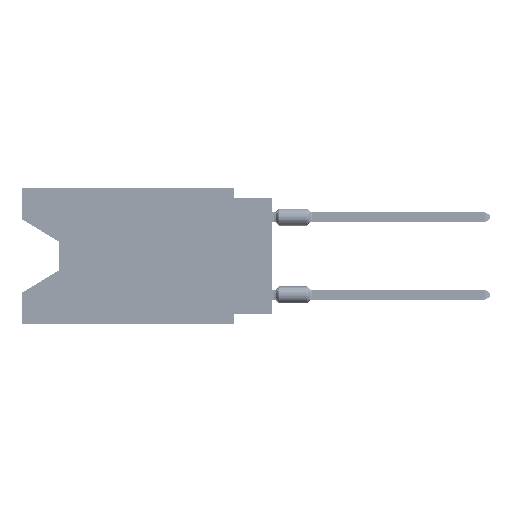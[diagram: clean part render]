
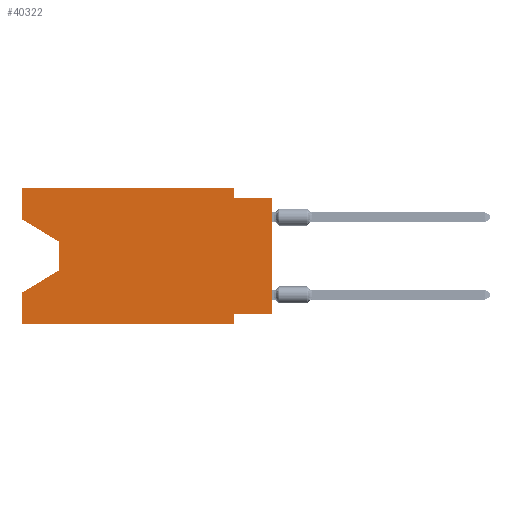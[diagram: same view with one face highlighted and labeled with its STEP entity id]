
A CAD part, left-side view. The second image highlights one B-rep face of the part: STEP entity #40322.
In plain terms, the highlighted planar face has unit normal (-1, 0, 0).
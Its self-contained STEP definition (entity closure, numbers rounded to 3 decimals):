
#5872 = VECTOR ( 'NONE', #108346, 1000. ) ;
#6425 = VECTOR ( 'NONE', #30490, 1000. ) ;
#6697 = ORIENTED_EDGE ( 'NONE', *, *, #8738, .T. ) ;
#8738 = EDGE_CURVE ( 'NONE', #48534, #78207, #15025, .T. ) ;
#10469 = LINE ( 'NONE', #19357, #81993 ) ;
#10480 = LINE ( 'NONE', #92791, #23293 ) ;
#11209 = ORIENTED_EDGE ( 'NONE', *, *, #109093, .F. ) ;
#12362 = CARTESIAN_POINT ( 'NONE',  ( 0., 13.97, -5.385 ) ) ;
#12400 = EDGE_CURVE ( 'NONE', #58064, #49808, #10480, .T. ) ;
#12422 = PLANE ( 'NONE',  #38660 ) ;
#14080 = CARTESIAN_POINT ( 'NONE',  ( 0., 16.383, 0. ) ) ;
#15025 = LINE ( 'NONE', #51156, #77540 ) ;
#15760 = EDGE_CURVE ( 'NONE', #78986, #49808, #52710, .T. ) ;
#15952 = CARTESIAN_POINT ( 'NONE',  ( 0., 0., -0.635 ) ) ;
#19357 = CARTESIAN_POINT ( 'NONE',  ( 0., 16.383, -2.038 ) ) ;
#20990 = ORIENTED_EDGE ( 'NONE', *, *, #60506, .F. ) ;
#23271 = ORIENTED_EDGE ( 'NONE', *, *, #80783, .F. ) ;
#23293 = VECTOR ( 'NONE', #46021, 1000. ) ;
#23773 = CARTESIAN_POINT ( 'NONE',  ( 0., 2.54, -8.255 ) ) ;
#24682 = DIRECTION ( 'NONE',  ( 0., 0., -1. ) ) ;
#24844 = CARTESIAN_POINT ( 'NONE',  ( 0., 16.383, 0. ) ) ;
#27945 = CARTESIAN_POINT ( 'NONE',  ( 0., 16.383, -8.89 ) ) ;
#30178 = ORIENTED_EDGE ( 'NONE', *, *, #110683, .T. ) ;
#30490 = DIRECTION ( 'NONE',  ( 0., 0., 1. ) ) ;
#30804 = CARTESIAN_POINT ( 'NONE',  ( 0., 16.383, 0. ) ) ;
#31590 = CARTESIAN_POINT ( 'NONE',  ( 0., 0., -0.635 ) ) ;
#32612 = CARTESIAN_POINT ( 'NONE',  ( 0., 13.97, -3.505 ) ) ;
#34746 = CARTESIAN_POINT ( 'NONE',  ( 0., 2.54, -0.635 ) ) ;
#35360 = CARTESIAN_POINT ( 'NONE',  ( 0., 16.383, 0. ) ) ;
#36560 = ORIENTED_EDGE ( 'NONE', *, *, #15760, .T. ) ;
#38660 = AXIS2_PLACEMENT_3D ( 'NONE', #48562, #68081, #59774 ) ;
#39693 = DIRECTION ( 'NONE',  ( 0., 0., 1. ) ) ;
#40322 = ADVANCED_FACE ( 'NONE', ( #40840 ), #12422, .F. ) ;
#40840 = FACE_OUTER_BOUND ( 'NONE', #113169, .T. ) ;
#43012 = VERTEX_POINT ( 'NONE', #34746 ) ;
#46021 = DIRECTION ( 'NONE',  ( 0., 0., -1. ) ) ;
#48250 = CARTESIAN_POINT ( 'NONE',  ( 0., 0., 0. ) ) ;
#48318 = ORIENTED_EDGE ( 'NONE', *, *, #92590, .T. ) ;
#48534 = VERTEX_POINT ( 'NONE', #12362 ) ;
#48562 = CARTESIAN_POINT ( 'NONE',  ( 0., 16.383, 0. ) ) ;
#48840 = LINE ( 'NONE', #48250, #6425 ) ;
#49808 = VERTEX_POINT ( 'NONE', #74140 ) ;
#51156 = CARTESIAN_POINT ( 'NONE',  ( 0., 13.97, -5.385 ) ) ;
#51755 = VECTOR ( 'NONE', #105972, 1000. ) ;
#52127 = CARTESIAN_POINT ( 'NONE',  ( 0., 16.383, -8.89 ) ) ;
#52710 = LINE ( 'NONE', #52127, #5872 ) ;
#55257 = VERTEX_POINT ( 'NONE', #88726 ) ;
#56885 = LINE ( 'NONE', #30804, #67182 ) ;
#58064 = VERTEX_POINT ( 'NONE', #23773 ) ;
#59415 = EDGE_CURVE ( 'NONE', #86997, #58064, #99359, .T. ) ;
#59774 = DIRECTION ( 'NONE',  ( 0., 0., -1. ) ) ;
#59967 = VECTOR ( 'NONE', #69463, 1000. ) ;
#60506 = EDGE_CURVE ( 'NONE', #83227, #55257, #70401, .T. ) ;
#63400 = ORIENTED_EDGE ( 'NONE', *, *, #116918, .F. ) ;
#64527 = DIRECTION ( 'NONE',  ( 0., 0., -1. ) ) ;
#66685 = CARTESIAN_POINT ( 'NONE',  ( 0., 16.383, -2.038 ) ) ;
#67182 = VECTOR ( 'NONE', #39693, 1000. ) ;
#67415 = EDGE_CURVE ( 'NONE', #86997, #109343, #48840, .T. ) ;
#68081 = DIRECTION ( 'NONE',  ( 1., 0., 0. ) ) ;
#68525 = CARTESIAN_POINT ( 'NONE',  ( 0., 16.383, -6.852 ) ) ;
#68759 = VERTEX_POINT ( 'NONE', #32612 ) ;
#69463 = DIRECTION ( 'NONE',  ( 0., -1., 0. ) ) ;
#69497 = DIRECTION ( 'NONE',  ( 0., 0.855, -0.519 ) ) ;
#69669 = LINE ( 'NONE', #105812, #97703 ) ;
#70401 = LINE ( 'NONE', #24844, #51755 ) ;
#71676 = VERTEX_POINT ( 'NONE', #66685 ) ;
#72810 = CARTESIAN_POINT ( 'NONE',  ( 0., 2.54, 0. ) ) ;
#74140 = CARTESIAN_POINT ( 'NONE',  ( 0., 2.54, -8.89 ) ) ;
#77540 = VECTOR ( 'NONE', #69497, 1000. ) ;
#78207 = VERTEX_POINT ( 'NONE', #68525 ) ;
#78986 = VERTEX_POINT ( 'NONE', #27945 ) ;
#80783 = EDGE_CURVE ( 'NONE', #43012, #109343, #87242, .T. ) ;
#81701 = LINE ( 'NONE', #72810, #115550 ) ;
#81993 = VECTOR ( 'NONE', #100505, 1000. ) ;
#83227 = VERTEX_POINT ( 'NONE', #35360 ) ;
#85185 = LINE ( 'NONE', #14080, #112044 ) ;
#86997 = VERTEX_POINT ( 'NONE', #110167 ) ;
#87242 = LINE ( 'NONE', #31590, #59967 ) ;
#88726 = CARTESIAN_POINT ( 'NONE',  ( 0., 2.54, 0. ) ) ;
#91033 = EDGE_CURVE ( 'NONE', #71676, #83227, #85185, .T. ) ;
#92262 = ORIENTED_EDGE ( 'NONE', *, *, #12400, .F. ) ;
#92590 = EDGE_CURVE ( 'NONE', #71676, #68759, #10469, .T. ) ;
#92791 = CARTESIAN_POINT ( 'NONE',  ( 0., 2.54, -8.89 ) ) ;
#94640 = DIRECTION ( 'NONE',  ( 0., 0., 1. ) ) ;
#97636 = ORIENTED_EDGE ( 'NONE', *, *, #67415, .T. ) ;
#97703 = VECTOR ( 'NONE', #24682, 1000. ) ;
#99359 = LINE ( 'NONE', #100556, #102561 ) ;
#100505 = DIRECTION ( 'NONE',  ( 0., -0.855, -0.519 ) ) ;
#100556 = CARTESIAN_POINT ( 'NONE',  ( 0., 0., -8.255 ) ) ;
#102302 = ORIENTED_EDGE ( 'NONE', *, *, #59415, .F. ) ;
#102561 = VECTOR ( 'NONE', #117169, 1000. ) ;
#105812 = CARTESIAN_POINT ( 'NONE',  ( 0., 13.97, -3.505 ) ) ;
#105972 = DIRECTION ( 'NONE',  ( 0., -1., 0. ) ) ;
#106776 = ORIENTED_EDGE ( 'NONE', *, *, #91033, .F. ) ;
#108346 = DIRECTION ( 'NONE',  ( 0., -1., 0. ) ) ;
#109093 = EDGE_CURVE ( 'NONE', #78986, #78207, #56885, .T. ) ;
#109343 = VERTEX_POINT ( 'NONE', #15952 ) ;
#110167 = CARTESIAN_POINT ( 'NONE',  ( 0., 0., -8.255 ) ) ;
#110683 = EDGE_CURVE ( 'NONE', #68759, #48534, #69669, .T. ) ;
#112044 = VECTOR ( 'NONE', #94640, 1000. ) ;
#113169 = EDGE_LOOP ( 'NONE', ( #48318, #30178, #6697, #11209, #36560, #92262, #102302, #97636, #23271, #63400, #20990, #106776 ) ) ;
#115550 = VECTOR ( 'NONE', #64527, 1000. ) ;
#116918 = EDGE_CURVE ( 'NONE', #55257, #43012, #81701, .T. ) ;
#117169 = DIRECTION ( 'NONE',  ( 0., 1., 0. ) ) ;
